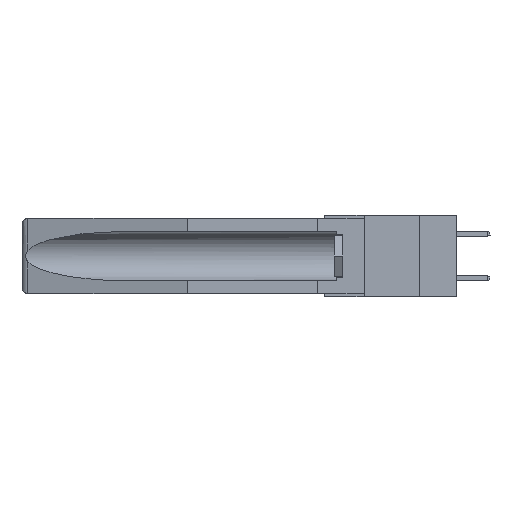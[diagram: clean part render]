
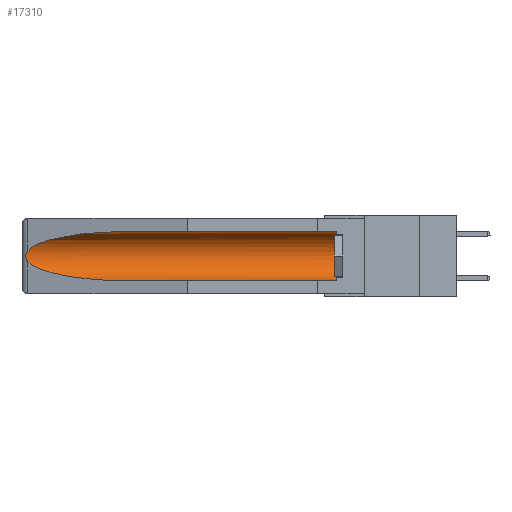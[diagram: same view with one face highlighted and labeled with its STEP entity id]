
A CAD part, left-side view. The second image highlights one B-rep face of the part: STEP entity #17310.
In plain terms, the highlighted cylindrical face has radius 2.857 mm (diameter 5.715 mm), a partial arc.
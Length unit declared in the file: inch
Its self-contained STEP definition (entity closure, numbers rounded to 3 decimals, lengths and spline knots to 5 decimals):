
#30 = EDGE_CURVE ( 'NONE', #8220, #18326, #10384, .T. ) ;
#178 = CARTESIAN_POINT ( 'NONE',  ( 0.26537, 1.52718, -0.14972 ) ) ;
#358 = CARTESIAN_POINT ( 'NONE',  ( 0.155, 0.126, -0.059 ) ) ;
#1203 = CARTESIAN_POINT ( 'NONE',  ( 0.26655, 1.53094, -0.18657 ) ) ;
#1501 = CARTESIAN_POINT ( 'NONE',  ( 0.155, 1.07973, -0.284 ) ) ;
#1775 = CARTESIAN_POINT ( 'NONE',  ( 0.25451, 1.48313, -0.09465 ) ) ;
#2381 = CARTESIAN_POINT ( 'NONE',  ( 0.155, 1.07973, -0.284 ) ) ;
#2402 = EDGE_CURVE ( 'NONE', #13616, #26162, #12317, .T. ) ;
#3137 =( BOUNDED_CURVE ( )  B_SPLINE_CURVE ( 3, ( #14851, #25618, #17276, #2381 ),
 .UNSPECIFIED., .F., .T. ) 
 B_SPLINE_CURVE_WITH_KNOTS ( ( 4, 4 ),
 ( 0.1948, 1.5708 ),
 .UNSPECIFIED. ) 
 CURVE ( )  GEOMETRIC_REPRESENTATION_ITEM ( )  RATIONAL_B_SPLINE_CURVE ( ( 1., 0.848, 0.848, 1. ) ) 
 REPRESENTATION_ITEM ( '' )  );
#3141 = ORIENTED_EDGE ( 'NONE', *, *, #30, .F. ) ;
#3448 = CARTESIAN_POINT ( 'NONE',  ( 0.26597, 1.52961, -0.15275 ) ) ;
#4989 = DIRECTION ( 'NONE',  ( 0., 1., 0. ) ) ;
#5255 = ORIENTED_EDGE ( 'NONE', *, *, #25970, .T. ) ;
#5503 = CARTESIAN_POINT ( 'NONE',  ( 0.2675, 1.53308, -0.16763 ) ) ;
#7516 = CARTESIAN_POINT ( 'NONE',  ( 0.2675, 1.53308, -0.17534 ) ) ;
#7607 = CARTESIAN_POINT ( 'NONE',  ( 0.26597, 1.5296, -0.19026 ) ) ;
#8076 = CARTESIAN_POINT ( 'NONE',  ( 0.21114, 1.30732, -0.059 ) ) ;
#8112 = ORIENTED_EDGE ( 'NONE', *, *, #13183, .T. ) ;
#8220 = VERTEX_POINT ( 'NONE', #24744 ) ;
#9390 = B_SPLINE_CURVE_WITH_KNOTS ( 'NONE', 3,
 ( #13886, #3448, #18039, #24637, #5503, #7516, #17954, #1203, #7607, #22433 ),
 .UNSPECIFIED., .F., .F.,
 ( 4, 2, 2, 2, 4 ),
 ( 0., 0.00029, 0.00058, 0.00087, 0.00117 ),
 .UNSPECIFIED. ) ;
#9691 = VECTOR ( 'NONE', #17191, 39.37008 ) ;
#10384 = LINE ( 'NONE', #12568, #9691 ) ;
#10837 = DIRECTION ( 'NONE',  ( 0., 0., 1. ) ) ;
#11215 = AXIS2_PLACEMENT_3D ( 'NONE', #17405, #12881, #10837 ) ;
#12317 =( BOUNDED_CURVE ( )  B_SPLINE_CURVE ( 3, ( #26849, #8076, #1775, #12413 ),
 .UNSPECIFIED., .F., .F. ) 
 B_SPLINE_CURVE_WITH_KNOTS ( ( 4, 4 ),
 ( 4.71239, 6.08839 ),
 .UNSPECIFIED. ) 
 CURVE ( )  GEOMETRIC_REPRESENTATION_ITEM ( )  RATIONAL_B_SPLINE_CURVE ( ( 1., 0.848, 0.848, 1. ) ) 
 REPRESENTATION_ITEM ( '' )  );
#12413 = CARTESIAN_POINT ( 'NONE',  ( 0.26537, 1.52718, -0.14972 ) ) ;
#12568 = CARTESIAN_POINT ( 'NONE',  ( 0.155, -0.30754, -0.284 ) ) ;
#12881 = DIRECTION ( 'NONE',  ( 0., -1., 0. ) ) ;
#13183 = EDGE_CURVE ( 'NONE', #27313, #13616, #15428, .T. ) ;
#13616 = VERTEX_POINT ( 'NONE', #16791 ) ;
#13886 = CARTESIAN_POINT ( 'NONE',  ( 0.26537, 1.52718, -0.14972 ) ) ;
#14816 = DIRECTION ( 'NONE',  ( 0., 1., 0. ) ) ;
#14851 = CARTESIAN_POINT ( 'NONE',  ( 0.26537, 1.52718, -0.19328 ) ) ;
#15428 = LINE ( 'NONE', #17456, #24068 ) ;
#16791 = CARTESIAN_POINT ( 'NONE',  ( 0.155, 1.07973, -0.059 ) ) ;
#17064 = ORIENTED_EDGE ( 'NONE', *, *, #2402, .T. ) ;
#17191 = DIRECTION ( 'NONE',  ( 0., 1., 0. ) ) ;
#17276 = CARTESIAN_POINT ( 'NONE',  ( 0.21114, 1.30732, -0.284 ) ) ;
#17310 = ADVANCED_FACE ( 'NONE', ( #26471 ), #19877, .F. ) ;
#17405 = CARTESIAN_POINT ( 'NONE',  ( 0.155, 0.126, -0.1715 ) ) ;
#17456 = CARTESIAN_POINT ( 'NONE',  ( 0.155, -0.30754, -0.059 ) ) ;
#17954 = CARTESIAN_POINT ( 'NONE',  ( 0.2673, 1.53269, -0.17917 ) ) ;
#18039 = CARTESIAN_POINT ( 'NONE',  ( 0.26654, 1.53092, -0.15636 ) ) ;
#18326 = VERTEX_POINT ( 'NONE', #1501 ) ;
#18341 = EDGE_CURVE ( 'NONE', #8220, #27313, #19482, .T. ) ;
#19010 = CARTESIAN_POINT ( 'NONE',  ( 0.26537, 1.52718, -0.19328 ) ) ;
#19023 = CARTESIAN_POINT ( 'NONE',  ( 0.155, -0.30754, -0.1715 ) ) ;
#19482 = CIRCLE ( 'NONE', #11215, 0.1125 ) ;
#19877 = CYLINDRICAL_SURFACE ( 'NONE', #21854, 0.1125 ) ;
#19991 = EDGE_CURVE ( 'NONE', #22045, #18326, #3137, .T. ) ;
#20814 = ORIENTED_EDGE ( 'NONE', *, *, #18341, .T. ) ;
#21854 = AXIS2_PLACEMENT_3D ( 'NONE', #19023, #14816, #23206 ) ;
#22045 = VERTEX_POINT ( 'NONE', #19010 ) ;
#22433 = CARTESIAN_POINT ( 'NONE',  ( 0.26537, 1.52718, -0.19328 ) ) ;
#23206 = DIRECTION ( 'NONE',  ( 0., 0., 1. ) ) ;
#23644 = EDGE_LOOP ( 'NONE', ( #17064, #5255, #25697, #3141, #20814, #8112 ) ) ;
#24068 = VECTOR ( 'NONE', #4989, 39.37008 ) ;
#24637 = CARTESIAN_POINT ( 'NONE',  ( 0.2673, 1.5327, -0.16383 ) ) ;
#24744 = CARTESIAN_POINT ( 'NONE',  ( 0.155, 0.126, -0.284 ) ) ;
#25618 = CARTESIAN_POINT ( 'NONE',  ( 0.25451, 1.48313, -0.24835 ) ) ;
#25697 = ORIENTED_EDGE ( 'NONE', *, *, #19991, .T. ) ;
#25970 = EDGE_CURVE ( 'NONE', #26162, #22045, #9390, .T. ) ;
#26162 = VERTEX_POINT ( 'NONE', #178 ) ;
#26471 = FACE_OUTER_BOUND ( 'NONE', #23644, .T. ) ;
#26849 = CARTESIAN_POINT ( 'NONE',  ( 0.155, 1.07973, -0.059 ) ) ;
#27313 = VERTEX_POINT ( 'NONE', #358 ) ;
